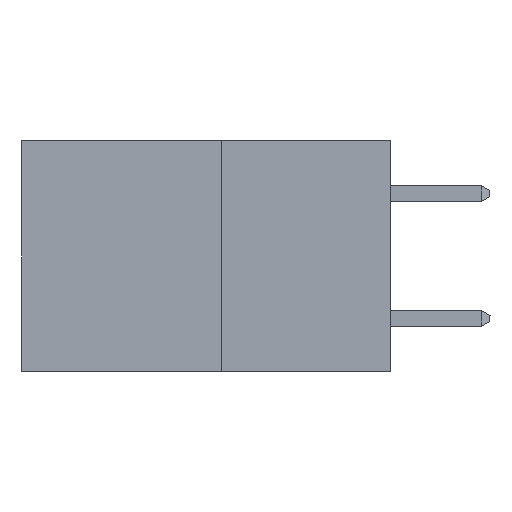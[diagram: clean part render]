
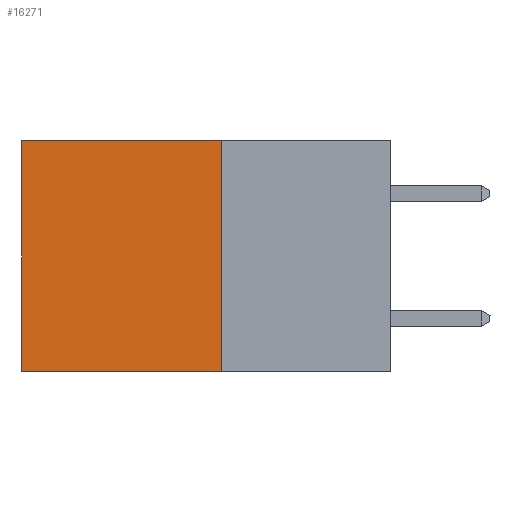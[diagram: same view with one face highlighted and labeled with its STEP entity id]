
A CAD part, left-side view. The second image highlights one B-rep face of the part: STEP entity #16271.
In plain terms, the highlighted planar face has unit normal (-1, 0, 0).
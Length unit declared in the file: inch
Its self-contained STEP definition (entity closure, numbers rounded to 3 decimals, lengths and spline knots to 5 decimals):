
#220 = EDGE_LOOP ( 'NONE', ( #10580, #20555, #2342, #19583 ) ) ;
#2072 = VERTEX_POINT ( 'NONE', #15151 ) ;
#2342 = ORIENTED_EDGE ( 'NONE', *, *, #11477, .F. ) ;
#2647 = EDGE_CURVE ( 'NONE', #2072, #4268, #14170, .T. ) ;
#2676 = VECTOR ( 'NONE', #19273, 39.37008 ) ;
#4268 = VERTEX_POINT ( 'NONE', #13892 ) ;
#4522 = PLANE ( 'NONE',  #17009 ) ;
#5321 = CARTESIAN_POINT ( 'NONE',  ( 0.277, 0.27, -0.37 ) ) ;
#6323 = CARTESIAN_POINT ( 'NONE',  ( 0.277, 0.27, -0.37 ) ) ;
#6332 = DIRECTION ( 'NONE',  ( 0., 0., -1. ) ) ;
#6420 = VECTOR ( 'NONE', #16587, 39.37008 ) ;
#6474 = CARTESIAN_POINT ( 'NONE',  ( 0.277, 0.59, -0.37 ) ) ;
#7201 = DIRECTION ( 'NONE',  ( 0., 1., 0. ) ) ;
#8072 = DIRECTION ( 'NONE',  ( 0., 0., -1. ) ) ;
#8194 = CARTESIAN_POINT ( 'NONE',  ( 0.277, 0.27, 0. ) ) ;
#9209 = VERTEX_POINT ( 'NONE', #18522 ) ;
#9926 = LINE ( 'NONE', #5321, #18338 ) ;
#10111 = VERTEX_POINT ( 'NONE', #14358 ) ;
#10580 = ORIENTED_EDGE ( 'NONE', *, *, #2647, .T. ) ;
#10943 = CARTESIAN_POINT ( 'NONE',  ( 0.277, 0.27, -0.37 ) ) ;
#11338 = EDGE_CURVE ( 'NONE', #10111, #4268, #9926, .T. ) ;
#11477 = EDGE_CURVE ( 'NONE', #9209, #10111, #16237, .T. ) ;
#11744 = EDGE_CURVE ( 'NONE', #9209, #2072, #19856, .T. ) ;
#13892 = CARTESIAN_POINT ( 'NONE',  ( 0.277, 0.59, -0.37 ) ) ;
#14170 = LINE ( 'NONE', #6474, #21503 ) ;
#14358 = CARTESIAN_POINT ( 'NONE',  ( 0.277, 0.27, -0.37 ) ) ;
#15151 = CARTESIAN_POINT ( 'NONE',  ( 0.277, 0.59, 0. ) ) ;
#16237 = LINE ( 'NONE', #10943, #2676 ) ;
#16271 = ADVANCED_FACE ( 'NONE', ( #17206 ), #4522, .F. ) ;
#16587 = DIRECTION ( 'NONE',  ( 0., 1., 0. ) ) ;
#17009 = AXIS2_PLACEMENT_3D ( 'NONE', #6323, #18146, #8072 ) ;
#17206 = FACE_OUTER_BOUND ( 'NONE', #220, .T. ) ;
#18146 = DIRECTION ( 'NONE',  ( 1., 0., 0. ) ) ;
#18338 = VECTOR ( 'NONE', #7201, 39.37008 ) ;
#18522 = CARTESIAN_POINT ( 'NONE',  ( 0.277, 0.27, 0. ) ) ;
#19273 = DIRECTION ( 'NONE',  ( 0., 0., -1. ) ) ;
#19583 = ORIENTED_EDGE ( 'NONE', *, *, #11744, .T. ) ;
#19856 = LINE ( 'NONE', #8194, #6420 ) ;
#20555 = ORIENTED_EDGE ( 'NONE', *, *, #11338, .F. ) ;
#21503 = VECTOR ( 'NONE', #6332, 39.37008 ) ;
